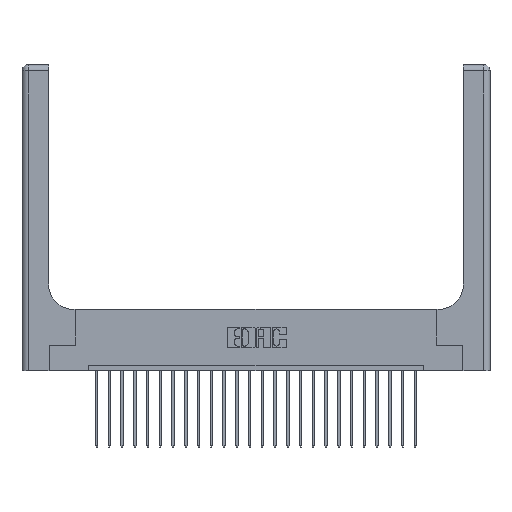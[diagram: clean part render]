
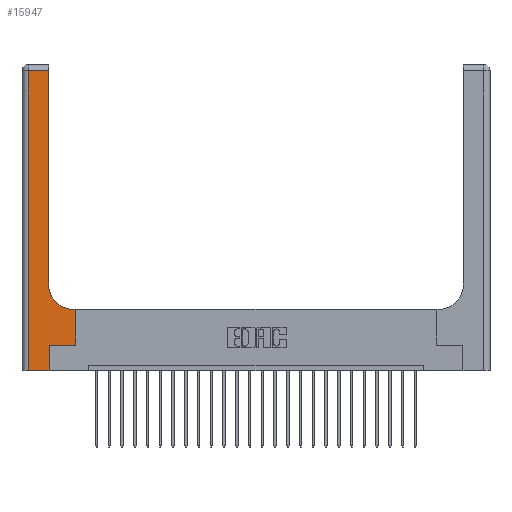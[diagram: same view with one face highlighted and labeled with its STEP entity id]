
A CAD part, top view. The second image highlights one B-rep face of the part: STEP entity #15947.
In plain terms, the highlighted planar face has unit normal (0, 0, 1).
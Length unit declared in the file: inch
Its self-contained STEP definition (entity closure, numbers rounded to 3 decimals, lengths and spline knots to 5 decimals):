
#116 = CARTESIAN_POINT ( 'NONE',  ( 0.265, 0., 0.37 ) ) ;
#999 = VECTOR ( 'NONE', #23347, 39.37008 ) ;
#1040 = CARTESIAN_POINT ( 'NONE',  ( 0.528, 0.25, 0.37 ) ) ;
#1147 = LINE ( 'NONE', #4898, #12741 ) ;
#1901 = VECTOR ( 'NONE', #4212, 39.37008 ) ;
#2743 = CARTESIAN_POINT ( 'NONE',  ( 0.26, 2.94, 0.37 ) ) ;
#3015 = CARTESIAN_POINT ( 'NONE',  ( 0.51, 0.6, 0.37 ) ) ;
#3177 = VECTOR ( 'NONE', #5103, 39.37008 ) ;
#3267 = CARTESIAN_POINT ( 'NONE',  ( 0.265, 0.25, 0.37 ) ) ;
#3329 = CARTESIAN_POINT ( 'NONE',  ( 0.26, 3., 0.37 ) ) ;
#3797 = LINE ( 'NONE', #3329, #5684 ) ;
#4212 = DIRECTION ( 'NONE',  ( 0., -1., 0. ) ) ;
#4408 = EDGE_LOOP ( 'NONE', ( #22134, #19773, #8982, #21341, #6166, #11811, #23434, #8030, #16390 ) ) ;
#4478 = VERTEX_POINT ( 'NONE', #21578 ) ;
#4685 = CIRCLE ( 'NONE', #8922, 0.25 ) ;
#4815 = CARTESIAN_POINT ( 'NONE',  ( 0.265, 0., 0.37 ) ) ;
#4898 = CARTESIAN_POINT ( 'NONE',  ( 0.528, 0.25, 0.37 ) ) ;
#4954 = EDGE_CURVE ( 'NONE', #4478, #12909, #7020, .T. ) ;
#5103 = DIRECTION ( 'NONE',  ( -1., 0., 0. ) ) ;
#5227 = PLANE ( 'NONE',  #17717 ) ;
#5372 = VERTEX_POINT ( 'NONE', #4815 ) ;
#5619 = DIRECTION ( 'NONE',  ( 0., 1., 0. ) ) ;
#5684 = VECTOR ( 'NONE', #10698, 39.37008 ) ;
#5686 = DIRECTION ( 'NONE',  ( 0., 1., 0. ) ) ;
#6166 = ORIENTED_EDGE ( 'NONE', *, *, #15126, .T. ) ;
#6546 = VERTEX_POINT ( 'NONE', #21657 ) ;
#7020 = LINE ( 'NONE', #12838, #3177 ) ;
#8030 = ORIENTED_EDGE ( 'NONE', *, *, #4954, .T. ) ;
#8866 = EDGE_CURVE ( 'NONE', #23460, #16554, #23470, .T. ) ;
#8922 = AXIS2_PLACEMENT_3D ( 'NONE', #15987, #16108, #14158 ) ;
#8982 = ORIENTED_EDGE ( 'NONE', *, *, #18358, .T. ) ;
#9194 = DIRECTION ( 'NONE',  ( -1., 0., 0. ) ) ;
#10067 = VECTOR ( 'NONE', #15621, 39.37008 ) ;
#10698 = DIRECTION ( 'NONE',  ( 0., 1., 0. ) ) ;
#10718 = VERTEX_POINT ( 'NONE', #11335 ) ;
#11335 = CARTESIAN_POINT ( 'NONE',  ( 0.06, 2.94, 0.37 ) ) ;
#11811 = ORIENTED_EDGE ( 'NONE', *, *, #8866, .T. ) ;
#11823 = CARTESIAN_POINT ( 'NONE',  ( 0.06, 3., 0.37 ) ) ;
#11858 = LINE ( 'NONE', #19234, #10067 ) ;
#12062 = LINE ( 'NONE', #11823, #1901 ) ;
#12244 = LINE ( 'NONE', #20110, #20603 ) ;
#12741 = VECTOR ( 'NONE', #5619, 39.37008 ) ;
#12838 = CARTESIAN_POINT ( 'NONE',  ( 0.26, 0.6, 0.37 ) ) ;
#12909 = VERTEX_POINT ( 'NONE', #3015 ) ;
#12999 = VERTEX_POINT ( 'NONE', #19591 ) ;
#13412 = VERTEX_POINT ( 'NONE', #2743 ) ;
#13750 = LINE ( 'NONE', #116, #20369 ) ;
#14095 = EDGE_CURVE ( 'NONE', #6546, #13412, #3797, .T. ) ;
#14158 = DIRECTION ( 'NONE',  ( 1., 0., 0. ) ) ;
#15126 = EDGE_CURVE ( 'NONE', #5372, #23460, #13750, .T. ) ;
#15621 = DIRECTION ( 'NONE',  ( 1., 0., 0. ) ) ;
#15947 = ADVANCED_FACE ( 'NONE', ( #23609 ), #5227, .F. ) ;
#15987 = CARTESIAN_POINT ( 'NONE',  ( 0.51, 0.85, 0.37 ) ) ;
#16108 = DIRECTION ( 'NONE',  ( 0., 0., -1. ) ) ;
#16390 = ORIENTED_EDGE ( 'NONE', *, *, #21091, .T. ) ;
#16554 = VERTEX_POINT ( 'NONE', #1040 ) ;
#17717 = AXIS2_PLACEMENT_3D ( 'NONE', #18175, #23732, #20444 ) ;
#18175 = CARTESIAN_POINT ( 'NONE',  ( 0., 3., 0.37 ) ) ;
#18358 = EDGE_CURVE ( 'NONE', #10718, #12999, #12062, .T. ) ;
#19077 = EDGE_CURVE ( 'NONE', #16554, #4478, #1147, .T. ) ;
#19234 = CARTESIAN_POINT ( 'NONE',  ( 0., 0., 0.37 ) ) ;
#19591 = CARTESIAN_POINT ( 'NONE',  ( 0.06, 0., 0.37 ) ) ;
#19773 = ORIENTED_EDGE ( 'NONE', *, *, #23294, .T. ) ;
#20110 = CARTESIAN_POINT ( 'NONE',  ( 0., 2.94, 0.37 ) ) ;
#20369 = VECTOR ( 'NONE', #5686, 39.37008 ) ;
#20444 = DIRECTION ( 'NONE',  ( -1., 0., 0. ) ) ;
#20603 = VECTOR ( 'NONE', #9194, 39.37008 ) ;
#21084 = EDGE_CURVE ( 'NONE', #12999, #5372, #11858, .T. ) ;
#21091 = EDGE_CURVE ( 'NONE', #12909, #6546, #4685, .T. ) ;
#21341 = ORIENTED_EDGE ( 'NONE', *, *, #21084, .T. ) ;
#21578 = CARTESIAN_POINT ( 'NONE',  ( 0.528, 0.6, 0.37 ) ) ;
#21657 = CARTESIAN_POINT ( 'NONE',  ( 0.26, 0.85, 0.37 ) ) ;
#22134 = ORIENTED_EDGE ( 'NONE', *, *, #14095, .T. ) ;
#22516 = CARTESIAN_POINT ( 'NONE',  ( 0.265, 0.25, 0.37 ) ) ;
#23294 = EDGE_CURVE ( 'NONE', #13412, #10718, #12244, .T. ) ;
#23347 = DIRECTION ( 'NONE',  ( 1., 0., 0. ) ) ;
#23434 = ORIENTED_EDGE ( 'NONE', *, *, #19077, .T. ) ;
#23460 = VERTEX_POINT ( 'NONE', #22516 ) ;
#23470 = LINE ( 'NONE', #3267, #999 ) ;
#23609 = FACE_OUTER_BOUND ( 'NONE', #4408, .T. ) ;
#23732 = DIRECTION ( 'NONE',  ( 0., 0., -1. ) ) ;
